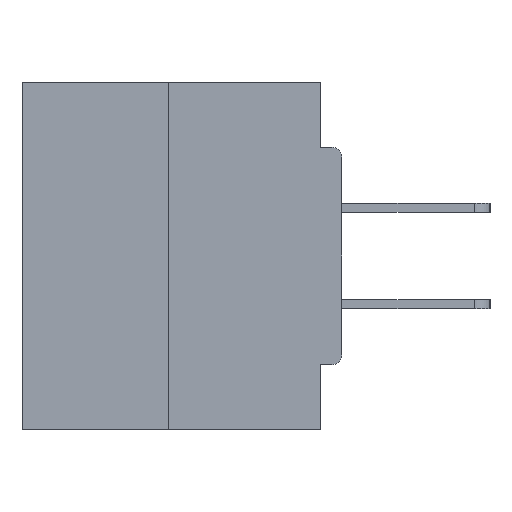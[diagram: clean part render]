
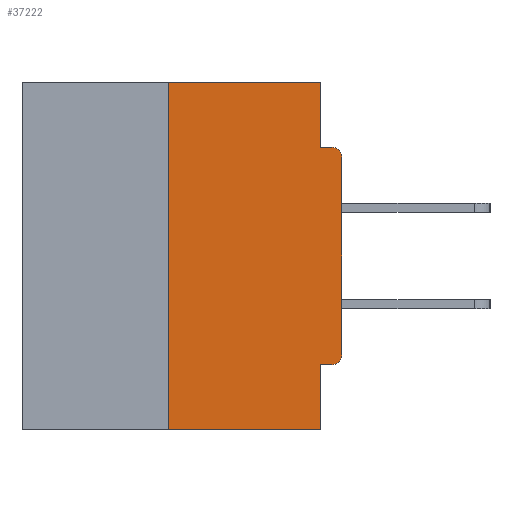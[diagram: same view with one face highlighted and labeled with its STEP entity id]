
A CAD part, left-side view. The second image highlights one B-rep face of the part: STEP entity #37222.
In plain terms, the highlighted planar face has unit normal (-1, 0, 0).
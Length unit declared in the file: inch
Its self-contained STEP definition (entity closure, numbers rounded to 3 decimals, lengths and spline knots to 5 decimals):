
#82 = DIRECTION ( 'NONE',  ( 1., 0., 0. ) ) ;
#205 = DIRECTION ( 'NONE',  ( 0., 0., -1. ) ) ;
#753 = LINE ( 'NONE', #25471, #28480 ) ;
#876 = CARTESIAN_POINT ( 'NONE',  ( 0., 0.031, -0.4065 ) ) ;
#1608 = DIRECTION ( 'NONE',  ( 0., 0., -1. ) ) ;
#1631 = EDGE_CURVE ( 'NONE', #12266, #33582, #14502, .T. ) ;
#1646 = VERTEX_POINT ( 'NONE', #30469 ) ;
#3151 = CARTESIAN_POINT ( 'NONE',  ( 0., 0.25, 0. ) ) ;
#4743 = ORIENTED_EDGE ( 'NONE', *, *, #14285, .T. ) ;
#6485 = ORIENTED_EDGE ( 'NONE', *, *, #28680, .T. ) ;
#6561 = VECTOR ( 'NONE', #39141, 39.37008 ) ;
#7608 = CARTESIAN_POINT ( 'NONE',  ( 0., 0.031, -0.0935 ) ) ;
#7900 = DIRECTION ( 'NONE',  ( 0., -1., 0. ) ) ;
#8569 = CARTESIAN_POINT ( 'NONE',  ( 0., 0.031, 0. ) ) ;
#8759 = EDGE_CURVE ( 'NONE', #31254, #1646, #20044, .T. ) ;
#9102 = CARTESIAN_POINT ( 'NONE',  ( 0., 0., -0.3915 ) ) ;
#9245 = VECTOR ( 'NONE', #27299, 39.37008 ) ;
#9601 = ORIENTED_EDGE ( 'NONE', *, *, #18693, .F. ) ;
#9851 = CARTESIAN_POINT ( 'NONE',  ( 0., 0.031, 0. ) ) ;
#10016 = CARTESIAN_POINT ( 'NONE',  ( 0., 0.031, -0.5 ) ) ;
#10773 = VECTOR ( 'NONE', #35498, 39.37008 ) ;
#11667 = ORIENTED_EDGE ( 'NONE', *, *, #1631, .F. ) ;
#11800 = VERTEX_POINT ( 'NONE', #10016 ) ;
#12048 = DIRECTION ( 'NONE',  ( -1., 0., 0. ) ) ;
#12266 = VERTEX_POINT ( 'NONE', #9851 ) ;
#12416 = CARTESIAN_POINT ( 'NONE',  ( 0., 0.015, -0.4065 ) ) ;
#13324 = DIRECTION ( 'NONE',  ( 0., 1., 0. ) ) ;
#13506 = LINE ( 'NONE', #30213, #9245 ) ;
#13706 = ORIENTED_EDGE ( 'NONE', *, *, #19330, .T. ) ;
#14038 = EDGE_CURVE ( 'NONE', #33582, #34054, #13506, .T. ) ;
#14285 = EDGE_CURVE ( 'NONE', #31254, #11800, #38367, .T. ) ;
#14502 = LINE ( 'NONE', #8569, #20706 ) ;
#14852 = CARTESIAN_POINT ( 'NONE',  ( 0., 0.46, 0. ) ) ;
#14921 = ORIENTED_EDGE ( 'NONE', *, *, #39217, .F. ) ;
#15661 = LINE ( 'NONE', #14852, #6561 ) ;
#16268 = VERTEX_POINT ( 'NONE', #35407 ) ;
#16885 = DIRECTION ( 'NONE',  ( -1., 0., 0. ) ) ;
#17538 = EDGE_LOOP ( 'NONE', ( #25251, #31021, #4743, #14921, #9601, #6485, #24134, #13706, #27402, #11667 ) ) ;
#17546 = VERTEX_POINT ( 'NONE', #12416 ) ;
#18541 = DIRECTION ( 'NONE',  ( 0., 0., 1. ) ) ;
#18693 = EDGE_CURVE ( 'NONE', #17546, #27451, #753, .T. ) ;
#18981 = EDGE_CURVE ( 'NONE', #26304, #16268, #19875, .T. ) ;
#19239 = VECTOR ( 'NONE', #7900, 39.37008 ) ;
#19330 = EDGE_CURVE ( 'NONE', #16268, #34054, #30746, .T. ) ;
#19405 = AXIS2_PLACEMENT_3D ( 'NONE', #21455, #82, #205 ) ;
#19875 = LINE ( 'NONE', #35627, #10773 ) ;
#20044 = LINE ( 'NONE', #3151, #26260 ) ;
#20126 = CARTESIAN_POINT ( 'NONE',  ( 0., 0.015, -0.0935 ) ) ;
#20706 = VECTOR ( 'NONE', #33125, 39.37008 ) ;
#21175 = PLANE ( 'NONE',  #19405 ) ;
#21264 = DIRECTION ( 'NONE',  ( 0., 0., -1. ) ) ;
#21455 = CARTESIAN_POINT ( 'NONE',  ( 0., 0.46, 0. ) ) ;
#22245 = DIRECTION ( 'NONE',  ( 0., 0., -1. ) ) ;
#24134 = ORIENTED_EDGE ( 'NONE', *, *, #18981, .T. ) ;
#24319 = LINE ( 'NONE', #24796, #25285 ) ;
#24796 = CARTESIAN_POINT ( 'NONE',  ( 0., 0.031, -0.5 ) ) ;
#24821 = AXIS2_PLACEMENT_3D ( 'NONE', #35184, #16885, #1608 ) ;
#25213 = CARTESIAN_POINT ( 'NONE',  ( 0., 0.25, -0.5 ) ) ;
#25251 = ORIENTED_EDGE ( 'NONE', *, *, #26197, .F. ) ;
#25285 = VECTOR ( 'NONE', #22245, 39.37008 ) ;
#25471 = CARTESIAN_POINT ( 'NONE',  ( 0., 0., -0.4065 ) ) ;
#26197 = EDGE_CURVE ( 'NONE', #1646, #12266, #15661, .T. ) ;
#26236 = CARTESIAN_POINT ( 'NONE',  ( 0., 0.46, -0.5 ) ) ;
#26260 = VECTOR ( 'NONE', #18541, 39.37008 ) ;
#26304 = VERTEX_POINT ( 'NONE', #9102 ) ;
#26610 = AXIS2_PLACEMENT_3D ( 'NONE', #30618, #12048, #21264 ) ;
#27299 = DIRECTION ( 'NONE',  ( 0., -1., 0. ) ) ;
#27402 = ORIENTED_EDGE ( 'NONE', *, *, #14038, .F. ) ;
#27451 = VERTEX_POINT ( 'NONE', #876 ) ;
#28480 = VECTOR ( 'NONE', #13324, 39.37008 ) ;
#28680 = EDGE_CURVE ( 'NONE', #17546, #26304, #29317, .T. ) ;
#29317 = CIRCLE ( 'NONE', #26610, 0.015 ) ;
#30213 = CARTESIAN_POINT ( 'NONE',  ( 0., 0., -0.0935 ) ) ;
#30469 = CARTESIAN_POINT ( 'NONE',  ( 0., 0.25, 0. ) ) ;
#30618 = CARTESIAN_POINT ( 'NONE',  ( 0., 0.015, -0.3915 ) ) ;
#30746 = CIRCLE ( 'NONE', #24821, 0.015 ) ;
#31021 = ORIENTED_EDGE ( 'NONE', *, *, #8759, .F. ) ;
#31254 = VERTEX_POINT ( 'NONE', #25213 ) ;
#33125 = DIRECTION ( 'NONE',  ( 0., 0., -1. ) ) ;
#33582 = VERTEX_POINT ( 'NONE', #7608 ) ;
#34054 = VERTEX_POINT ( 'NONE', #20126 ) ;
#35184 = CARTESIAN_POINT ( 'NONE',  ( 0., 0.015, -0.1085 ) ) ;
#35407 = CARTESIAN_POINT ( 'NONE',  ( 0., 0., -0.1085 ) ) ;
#35498 = DIRECTION ( 'NONE',  ( 0., 0., 1. ) ) ;
#35627 = CARTESIAN_POINT ( 'NONE',  ( 0., 0., 0. ) ) ;
#36533 = FACE_OUTER_BOUND ( 'NONE', #17538, .T. ) ;
#37222 = ADVANCED_FACE ( 'NONE', ( #36533 ), #21175, .F. ) ;
#38367 = LINE ( 'NONE', #26236, #19239 ) ;
#39141 = DIRECTION ( 'NONE',  ( 0., -1., 0. ) ) ;
#39217 = EDGE_CURVE ( 'NONE', #27451, #11800, #24319, .T. ) ;
